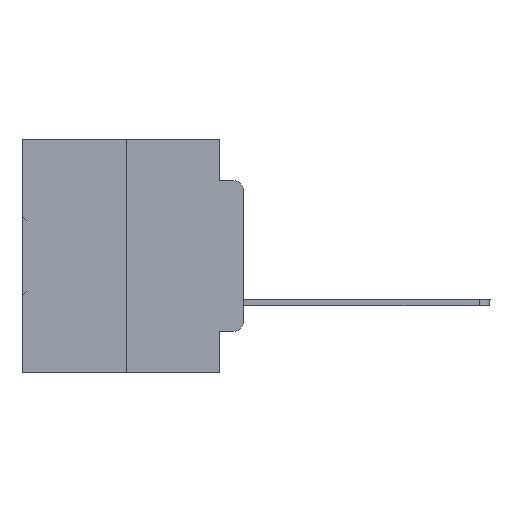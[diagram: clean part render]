
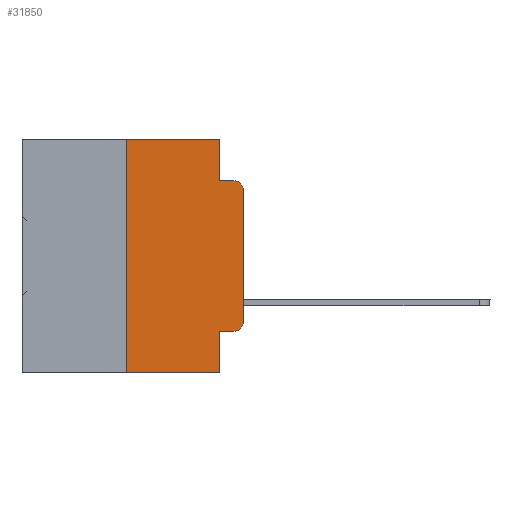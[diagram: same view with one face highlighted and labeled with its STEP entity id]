
A CAD part, left-side view. The second image highlights one B-rep face of the part: STEP entity #31850.
In plain terms, the highlighted planar face has unit normal (-1, 0, 0).
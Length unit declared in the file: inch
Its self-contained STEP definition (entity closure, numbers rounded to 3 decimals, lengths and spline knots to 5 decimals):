
#105 = EDGE_CURVE ( 'NONE', #6097, #6269, #7399, .T. ) ;
#378 = CARTESIAN_POINT ( 'NONE',  ( 0., 0.051, 0. ) ) ;
#798 = CARTESIAN_POINT ( 'NONE',  ( 0., 0., -0.3915 ) ) ;
#840 = CARTESIAN_POINT ( 'NONE',  ( 0., 0.473, 0. ) ) ;
#927 = VECTOR ( 'NONE', #8266, 39.37008 ) ;
#1167 = VERTEX_POINT ( 'NONE', #378 ) ;
#1393 = LINE ( 'NONE', #8594, #927 ) ;
#2328 = DIRECTION ( 'NONE',  ( 0., 0., 1. ) ) ;
#2963 = CARTESIAN_POINT ( 'NONE',  ( 0., 0.02, -0.4115 ) ) ;
#3065 = EDGE_CURVE ( 'NONE', #10793, #6097, #11873, .T. ) ;
#3463 = VECTOR ( 'NONE', #29401, 39.37008 ) ;
#3548 = EDGE_CURVE ( 'NONE', #6269, #15626, #34776, .T. ) ;
#3676 = VERTEX_POINT ( 'NONE', #22336 ) ;
#4520 = LINE ( 'NONE', #33170, #22825 ) ;
#5225 = DIRECTION ( 'NONE',  ( 0., -1., 0. ) ) ;
#6097 = VERTEX_POINT ( 'NONE', #2963 ) ;
#6269 = VERTEX_POINT ( 'NONE', #798 ) ;
#6356 = VERTEX_POINT ( 'NONE', #26044 ) ;
#6408 = EDGE_CURVE ( 'NONE', #15626, #22103, #9489, .T. ) ;
#7399 = CIRCLE ( 'NONE', #13260, 0.02 ) ;
#8160 = CARTESIAN_POINT ( 'NONE',  ( 0., 0.473, -0.5 ) ) ;
#8266 = DIRECTION ( 'NONE',  ( 0., -1., 0. ) ) ;
#8515 = ORIENTED_EDGE ( 'NONE', *, *, #9057, .F. ) ;
#8594 = CARTESIAN_POINT ( 'NONE',  ( 0., 0.473, 0. ) ) ;
#8794 = CARTESIAN_POINT ( 'NONE',  ( 0., 0.051, -0.4115 ) ) ;
#9057 = EDGE_CURVE ( 'NONE', #31439, #22103, #26258, .T. ) ;
#9489 = CIRCLE ( 'NONE', #15806, 0.02 ) ;
#9616 = CARTESIAN_POINT ( 'NONE',  ( 0., 0.051, -0.0885 ) ) ;
#9617 = DIRECTION ( 'NONE',  ( -1., 0., 0. ) ) ;
#9677 = VECTOR ( 'NONE', #5225, 39.37008 ) ;
#10793 = VERTEX_POINT ( 'NONE', #23557 ) ;
#11255 = CARTESIAN_POINT ( 'NONE',  ( 0., 0.02, -0.0885 ) ) ;
#11428 = ORIENTED_EDGE ( 'NONE', *, *, #25973, .F. ) ;
#11536 = ORIENTED_EDGE ( 'NONE', *, *, #19831, .F. ) ;
#11827 = DIRECTION ( 'NONE',  ( 1., 0., 0. ) ) ;
#11873 = LINE ( 'NONE', #8794, #25447 ) ;
#13260 = AXIS2_PLACEMENT_3D ( 'NONE', #32021, #29386, #32274 ) ;
#14927 = ORIENTED_EDGE ( 'NONE', *, *, #3065, .T. ) ;
#15059 = DIRECTION ( 'NONE',  ( 0., 0., -1. ) ) ;
#15626 = VERTEX_POINT ( 'NONE', #34246 ) ;
#15806 = AXIS2_PLACEMENT_3D ( 'NONE', #20608, #9617, #34114 ) ;
#16931 = ORIENTED_EDGE ( 'NONE', *, *, #3548, .T. ) ;
#17210 = FACE_OUTER_BOUND ( 'NONE', #22296, .T. ) ;
#19408 = DIRECTION ( 'NONE',  ( 0., 0., 1. ) ) ;
#19490 = VECTOR ( 'NONE', #19408, 39.37008 ) ;
#19617 = VECTOR ( 'NONE', #22808, 39.37008 ) ;
#19736 = EDGE_CURVE ( 'NONE', #6356, #3676, #25193, .T. ) ;
#19769 = EDGE_CURVE ( 'NONE', #6356, #34181, #21464, .T. ) ;
#19831 = EDGE_CURVE ( 'NONE', #34181, #1167, #1393, .T. ) ;
#20488 = AXIS2_PLACEMENT_3D ( 'NONE', #840, #11827, #15059 ) ;
#20608 = CARTESIAN_POINT ( 'NONE',  ( 0., 0.02, -0.1085 ) ) ;
#21338 = CARTESIAN_POINT ( 'NONE',  ( 0., 0.051, -0.0885 ) ) ;
#21464 = LINE ( 'NONE', #27169, #31553 ) ;
#21698 = ORIENTED_EDGE ( 'NONE', *, *, #19736, .T. ) ;
#22103 = VERTEX_POINT ( 'NONE', #11255 ) ;
#22296 = EDGE_LOOP ( 'NONE', ( #16931, #29807, #8515, #11428, #11536, #35176, #21698, #26153, #14927, #23790 ) ) ;
#22336 = CARTESIAN_POINT ( 'NONE',  ( 0., 0.051, -0.5 ) ) ;
#22508 = PLANE ( 'NONE',  #20488 ) ;
#22808 = DIRECTION ( 'NONE',  ( 0., 0., -1. ) ) ;
#22825 = VECTOR ( 'NONE', #30365, 39.37008 ) ;
#23557 = CARTESIAN_POINT ( 'NONE',  ( 0., 0.051, -0.4115 ) ) ;
#23790 = ORIENTED_EDGE ( 'NONE', *, *, #105, .T. ) ;
#24505 = CARTESIAN_POINT ( 'NONE',  ( 0., 0., 0. ) ) ;
#25193 = LINE ( 'NONE', #8160, #3463 ) ;
#25447 = VECTOR ( 'NONE', #33301, 39.37008 ) ;
#25973 = EDGE_CURVE ( 'NONE', #1167, #31439, #4520, .T. ) ;
#26044 = CARTESIAN_POINT ( 'NONE',  ( 0., 0.25, -0.5 ) ) ;
#26153 = ORIENTED_EDGE ( 'NONE', *, *, #28145, .F. ) ;
#26258 = LINE ( 'NONE', #21338, #9677 ) ;
#27169 = CARTESIAN_POINT ( 'NONE',  ( 0., 0.25, 0. ) ) ;
#28145 = EDGE_CURVE ( 'NONE', #10793, #3676, #32787, .T. ) ;
#29386 = DIRECTION ( 'NONE',  ( -1., 0., 0. ) ) ;
#29401 = DIRECTION ( 'NONE',  ( 0., -1., 0. ) ) ;
#29807 = ORIENTED_EDGE ( 'NONE', *, *, #6408, .T. ) ;
#30365 = DIRECTION ( 'NONE',  ( 0., 0., -1. ) ) ;
#31439 = VERTEX_POINT ( 'NONE', #9616 ) ;
#31553 = VECTOR ( 'NONE', #2328, 39.37008 ) ;
#31850 = ADVANCED_FACE ( 'NONE', ( #17210 ), #22508, .F. ) ;
#32021 = CARTESIAN_POINT ( 'NONE',  ( 0., 0.02, -0.3915 ) ) ;
#32274 = DIRECTION ( 'NONE',  ( 0., 0., -1. ) ) ;
#32787 = LINE ( 'NONE', #33848, #19617 ) ;
#33170 = CARTESIAN_POINT ( 'NONE',  ( 0., 0.051, 0. ) ) ;
#33301 = DIRECTION ( 'NONE',  ( 0., -1., 0. ) ) ;
#33848 = CARTESIAN_POINT ( 'NONE',  ( 0., 0.051, 0. ) ) ;
#34114 = DIRECTION ( 'NONE',  ( 0., 0., -1. ) ) ;
#34181 = VERTEX_POINT ( 'NONE', #34541 ) ;
#34246 = CARTESIAN_POINT ( 'NONE',  ( 0., 0., -0.1085 ) ) ;
#34541 = CARTESIAN_POINT ( 'NONE',  ( 0., 0.25, 0. ) ) ;
#34776 = LINE ( 'NONE', #24505, #19490 ) ;
#35176 = ORIENTED_EDGE ( 'NONE', *, *, #19769, .F. ) ;
